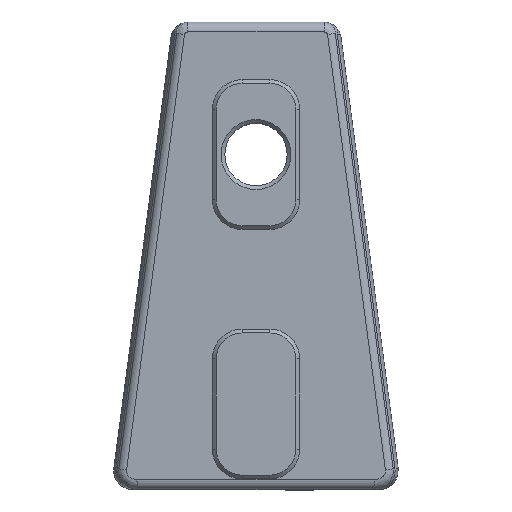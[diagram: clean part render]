
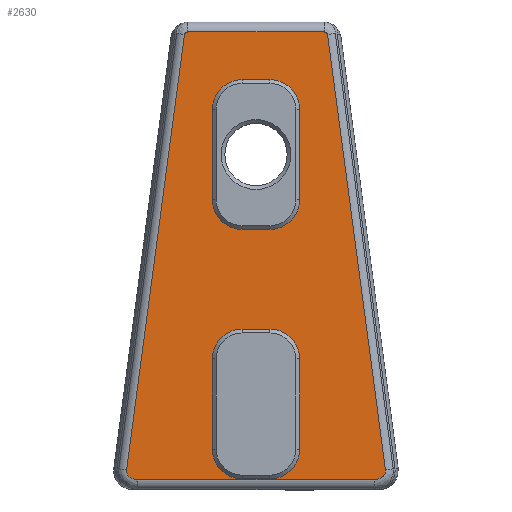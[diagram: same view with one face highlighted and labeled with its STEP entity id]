
A CAD part, top view. The second image highlights one B-rep face of the part: STEP entity #2630.
In plain terms, the highlighted planar face has unit normal (0, 0, 1).
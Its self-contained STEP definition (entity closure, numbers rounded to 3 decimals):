
#30=ELLIPSE('',#2906,0.891,0.7);
#32=ELLIPSE('',#2914,0.891,0.7);
#50=FACE_BOUND('',#581,.T.);
#51=FACE_BOUND('',#582,.T.);
#114=PLANE('',#2922);
#180=B_SPLINE_CURVE_WITH_KNOTS('',3,(#5896,#5897,#5898,#5899,#5900),
 .UNSPECIFIED.,.F.,.F.,(4,1,4),(0.,0.015,0.035),
 .UNSPECIFIED.);
#182=B_SPLINE_CURVE_WITH_KNOTS('',3,(#5992,#5993,#5994,#5995,#5996),
 .UNSPECIFIED.,.F.,.F.,(4,1,4),(0.,0.02,
0.035),.UNSPECIFIED.);
#396=FACE_OUTER_BOUND('',#580,.T.);
#580=EDGE_LOOP('',(#2281,#2282,#2283,#2284,#2285,#2286,#2287,#2288));
#581=EDGE_LOOP('',(#2289,#2290,#2291,#2292,#2293,#2294,#2295,#2296));
#582=EDGE_LOOP('',(#2297,#2298,#2299,#2300,#2301,#2302,#2303,#2304));
#660=LINE('',#4290,#814);
#663=LINE('',#4298,#817);
#683=LINE('',#4356,#837);
#686=LINE('',#4364,#840);
#693=LINE('',#4387,#847);
#694=LINE('',#4389,#848);
#749=LINE('',#5906,#903);
#750=LINE('',#5944,#904);
#751=LINE('',#5950,#905);
#754=LINE('',#6031,#908);
#758=LINE('',#6050,#912);
#759=LINE('',#6051,#913);
#814=VECTOR('',#3131,10.);
#817=VECTOR('',#3140,10.);
#837=VECTOR('',#3198,10.);
#840=VECTOR('',#3207,10.);
#847=VECTOR('',#3234,10.);
#848=VECTOR('',#3237,10.);
#903=VECTOR('',#3558,10.);
#904=VECTOR('',#3569,10.);
#905=VECTOR('',#3574,10.);
#908=VECTOR('',#3587,10.);
#912=VECTOR('',#3605,10.);
#913=VECTOR('',#3606,10.);
#952=CIRCLE('',#2733,2.38);
#953=CIRCLE('',#2736,2.38);
#962=CIRCLE('',#2755,2.38);
#963=CIRCLE('',#2758,2.38);
#964=CIRCLE('',#2762,2.38);
#965=CIRCLE('',#2764,2.38);
#966=CIRCLE('',#2766,2.38);
#967=CIRCLE('',#2768,2.38);
#1118=VERTEX_POINT('',#4282);
#1119=VERTEX_POINT('',#4284);
#1120=VERTEX_POINT('',#4288);
#1121=VERTEX_POINT('',#4292);
#1122=VERTEX_POINT('',#4296);
#1139=VERTEX_POINT('',#4348);
#1140=VERTEX_POINT('',#4350);
#1141=VERTEX_POINT('',#4354);
#1142=VERTEX_POINT('',#4358);
#1143=VERTEX_POINT('',#4362);
#1144=VERTEX_POINT('',#4367);
#1145=VERTEX_POINT('',#4369);
#1146=VERTEX_POINT('',#4373);
#1147=VERTEX_POINT('',#4377);
#1148=VERTEX_POINT('',#4379);
#1149=VERTEX_POINT('',#4383);
#1238=VERTEX_POINT('',#5885);
#1241=VERTEX_POINT('',#5894);
#1242=VERTEX_POINT('',#5902);
#1244=VERTEX_POINT('',#5937);
#1245=VERTEX_POINT('',#5942);
#1247=VERTEX_POINT('',#5947);
#1248=VERTEX_POINT('',#5949);
#1250=VERTEX_POINT('',#5984);
#1373=EDGE_CURVE('',#1119,#1118,#952,.T.);
#1376=EDGE_CURVE('',#1118,#1120,#660,.T.);
#1378=EDGE_CURVE('',#1120,#1121,#953,.T.);
#1380=EDGE_CURVE('',#1121,#1122,#663,.F.);
#1406=EDGE_CURVE('',#1139,#1140,#962,.T.);
#1409=EDGE_CURVE('',#1141,#1139,#683,.T.);
#1411=EDGE_CURVE('',#1142,#1141,#963,.T.);
#1413=EDGE_CURVE('',#1142,#1143,#686,.F.);
#1415=EDGE_CURVE('',#1144,#1145,#964,.T.);
#1418=EDGE_CURVE('',#1146,#1122,#965,.T.);
#1420=EDGE_CURVE('',#1148,#1147,#966,.T.);
#1423=EDGE_CURVE('',#1143,#1149,#967,.T.);
#1424=EDGE_CURVE('',#1145,#1146,#693,.T.);
#1425=EDGE_CURVE('',#1149,#1148,#694,.T.);
#1586=EDGE_CURVE('',#1241,#1238,#180,.T.);
#1589=EDGE_CURVE('',#1238,#1242,#749,.T.);
#1592=EDGE_CURVE('',#1242,#1244,#30,.T.);
#1594=EDGE_CURVE('',#1244,#1245,#750,.T.);
#1596=EDGE_CURVE('',#1247,#1248,#751,.T.);
#1601=EDGE_CURVE('',#1248,#1250,#182,.T.);
#1603=EDGE_CURVE('',#1245,#1247,#32,.T.);
#1605=EDGE_CURVE('',#1250,#1241,#754,.T.);
#1613=EDGE_CURVE('',#1140,#1147,#758,.T.);
#1614=EDGE_CURVE('',#1119,#1144,#759,.T.);
#2281=ORIENTED_EDGE('',*,*,#1596,.F.);
#2282=ORIENTED_EDGE('',*,*,#1603,.F.);
#2283=ORIENTED_EDGE('',*,*,#1594,.F.);
#2284=ORIENTED_EDGE('',*,*,#1592,.F.);
#2285=ORIENTED_EDGE('',*,*,#1589,.F.);
#2286=ORIENTED_EDGE('',*,*,#1586,.F.);
#2287=ORIENTED_EDGE('',*,*,#1605,.F.);
#2288=ORIENTED_EDGE('',*,*,#1601,.F.);
#2289=ORIENTED_EDGE('',*,*,#1413,.T.);
#2290=ORIENTED_EDGE('',*,*,#1423,.T.);
#2291=ORIENTED_EDGE('',*,*,#1425,.T.);
#2292=ORIENTED_EDGE('',*,*,#1420,.T.);
#2293=ORIENTED_EDGE('',*,*,#1613,.F.);
#2294=ORIENTED_EDGE('',*,*,#1406,.F.);
#2295=ORIENTED_EDGE('',*,*,#1409,.F.);
#2296=ORIENTED_EDGE('',*,*,#1411,.F.);
#2297=ORIENTED_EDGE('',*,*,#1418,.F.);
#2298=ORIENTED_EDGE('',*,*,#1424,.F.);
#2299=ORIENTED_EDGE('',*,*,#1415,.F.);
#2300=ORIENTED_EDGE('',*,*,#1614,.F.);
#2301=ORIENTED_EDGE('',*,*,#1373,.T.);
#2302=ORIENTED_EDGE('',*,*,#1376,.T.);
#2303=ORIENTED_EDGE('',*,*,#1378,.T.);
#2304=ORIENTED_EDGE('',*,*,#1380,.T.);
#2630=ADVANCED_FACE('',(#396,#50,#51),#114,.F.);
#2733=AXIS2_PLACEMENT_3D('',#4285,#3125,#3126);
#2736=AXIS2_PLACEMENT_3D('',#4294,#3135,#3136);
#2755=AXIS2_PLACEMENT_3D('',#4351,#3192,#3193);
#2758=AXIS2_PLACEMENT_3D('',#4360,#3202,#3203);
#2762=AXIS2_PLACEMENT_3D('',#4370,#3213,#3214);
#2764=AXIS2_PLACEMENT_3D('',#4375,#3219,#3220);
#2766=AXIS2_PLACEMENT_3D('',#4380,#3224,#3225);
#2768=AXIS2_PLACEMENT_3D('',#4385,#3230,#3231);
#2906=AXIS2_PLACEMENT_3D('',#5940,#3563,#3564);
#2914=AXIS2_PLACEMENT_3D('',#6028,#3582,#3583);
#2922=AXIS2_PLACEMENT_3D('',#6049,#3603,#3604);
#3125=DIRECTION('center_axis',(0.,0.,-1.));
#3126=DIRECTION('ref_axis',(0.,1.,0.));
#3131=DIRECTION('',(1.,0.,0.));
#3135=DIRECTION('center_axis',(0.,0.,-1.));
#3136=DIRECTION('ref_axis',(1.,0.,0.));
#3140=DIRECTION('',(0.,1.,0.));
#3192=DIRECTION('center_axis',(0.,0.,1.));
#3193=DIRECTION('ref_axis',(0.,1.,0.));
#3198=DIRECTION('',(-1.,0.,0.));
#3202=DIRECTION('center_axis',(0.,0.,1.));
#3203=DIRECTION('ref_axis',(1.,0.,0.));
#3207=DIRECTION('',(0.,1.,0.));
#3213=DIRECTION('center_axis',(0.,0.,1.));
#3214=DIRECTION('ref_axis',(-1.,0.,0.));
#3219=DIRECTION('center_axis',(0.,0.,1.));
#3220=DIRECTION('ref_axis',(0.,-1.,0.));
#3224=DIRECTION('center_axis',(0.,0.,-1.));
#3225=DIRECTION('ref_axis',(-1.,0.,0.));
#3230=DIRECTION('center_axis',(0.,0.,-1.));
#3231=DIRECTION('ref_axis',(0.,-1.,0.));
#3234=DIRECTION('',(1.,0.,0.));
#3237=DIRECTION('',(-1.,0.,0.));
#3558=DIRECTION('',(0.132,-0.991,0.));
#3563=DIRECTION('center_axis',(0.,0.,-1.));
#3564=DIRECTION('ref_axis',(1.,0.,0.));
#3569=DIRECTION('',(-1.,0.,0.));
#3574=DIRECTION('',(0.132,0.991,0.));
#3582=DIRECTION('center_axis',(0.,0.,-1.));
#3583=DIRECTION('ref_axis',(-1.,0.,0.));
#3587=DIRECTION('',(1.,0.,0.));
#3603=DIRECTION('center_axis',(0.,0.,-1.));
#3604=DIRECTION('ref_axis',(1.,0.,0.));
#3605=DIRECTION('',(0.,-1.,0.));
#3606=DIRECTION('',(0.,-1.,0.));
#4282=CARTESIAN_POINT('',(-1.12,39.1,-1.));
#4284=CARTESIAN_POINT('',(-3.5,36.72,-1.));
#4285=CARTESIAN_POINT('Origin',(-1.12,36.72,-1.));
#4288=CARTESIAN_POINT('',(1.12,39.1,-1.));
#4290=CARTESIAN_POINT('',(-0.56,39.1,-1.));
#4292=CARTESIAN_POINT('',(3.5,36.72,-1.));
#4294=CARTESIAN_POINT('Origin',(1.12,36.72,-1.));
#4296=CARTESIAN_POINT('',(3.5,29.48,-1.));
#4298=CARTESIAN_POINT('',(3.5,5.35,-1.));
#4348=CARTESIAN_POINT('',(-1.12,19.1,-1.));
#4350=CARTESIAN_POINT('',(-3.5,16.72,-1.));
#4351=CARTESIAN_POINT('Origin',(-1.12,16.72,-1.));
#4354=CARTESIAN_POINT('',(1.12,19.1,-1.));
#4356=CARTESIAN_POINT('',(0.56,19.1,-1.));
#4358=CARTESIAN_POINT('',(3.5,16.72,-1.));
#4360=CARTESIAN_POINT('Origin',(1.12,16.72,-1.));
#4362=CARTESIAN_POINT('',(3.5,9.48,-1.));
#4364=CARTESIAN_POINT('',(3.5,5.35,-1.));
#4367=CARTESIAN_POINT('',(-3.5,29.48,-1.));
#4369=CARTESIAN_POINT('',(-1.12,27.1,-1.));
#4370=CARTESIAN_POINT('Origin',(-1.12,29.48,-1.));
#4373=CARTESIAN_POINT('',(1.12,27.1,-1.));
#4375=CARTESIAN_POINT('Origin',(1.12,29.48,-1.));
#4377=CARTESIAN_POINT('',(-3.5,9.48,-1.));
#4379=CARTESIAN_POINT('',(-1.12,7.1,-1.));
#4380=CARTESIAN_POINT('Origin',(-1.12,9.48,-1.));
#4383=CARTESIAN_POINT('',(1.12,7.1,-1.));
#4385=CARTESIAN_POINT('Origin',(1.12,9.48,-1.));
#4387=CARTESIAN_POINT('',(-0.56,27.1,-1.));
#4389=CARTESIAN_POINT('',(0.56,7.1,-1.));
#5885=CARTESIAN_POINT('',(5.733,42.73,-1.));
#5894=CARTESIAN_POINT('',(5.473,42.928,-1.));
#5896=CARTESIAN_POINT('Ctrl Pts',(5.473,42.928,-1.));
#5897=CARTESIAN_POINT('Ctrl Pts',(5.524,42.928,-1.));
#5898=CARTESIAN_POINT('Ctrl Pts',(5.64,42.896,-1.));
#5899=CARTESIAN_POINT('Ctrl Pts',(5.724,42.797,-1.));
#5900=CARTESIAN_POINT('Ctrl Pts',(5.733,42.73,-1.));
#5902=CARTESIAN_POINT('',(10.371,7.823,-1.));
#5906=CARTESIAN_POINT('',(7.54,29.131,-1.));
#5937=CARTESIAN_POINT('',(9.485,7.05,-1.));
#5940=CARTESIAN_POINT('Origin',(9.485,7.75,-1.));
#5942=CARTESIAN_POINT('',(-9.485,7.05,-1.));
#5944=CARTESIAN_POINT('',(0.56,7.05,-1.));
#5947=CARTESIAN_POINT('',(-10.371,7.823,-1.));
#5949=CARTESIAN_POINT('',(-5.733,42.73,-1.));
#5950=CARTESIAN_POINT('',(-8.719,20.256,-1.));
#5984=CARTESIAN_POINT('',(-5.473,42.928,-1.));
#5992=CARTESIAN_POINT('Ctrl Pts',(-5.733,42.73,-1.));
#5993=CARTESIAN_POINT('Ctrl Pts',(-5.724,42.797,-1.));
#5994=CARTESIAN_POINT('Ctrl Pts',(-5.64,42.896,-1.));
#5995=CARTESIAN_POINT('Ctrl Pts',(-5.524,42.928,-1.));
#5996=CARTESIAN_POINT('Ctrl Pts',(-5.473,42.928,-1.));
#6028=CARTESIAN_POINT('Origin',(-9.485,7.75,-1.));
#6031=CARTESIAN_POINT('',(0.,42.928,-1.));
#6049=CARTESIAN_POINT('Origin',(0.,24.,-1.));
#6050=CARTESIAN_POINT('',(-3.5,5.35,-1.));
#6051=CARTESIAN_POINT('',(-3.5,5.35,-1.));
